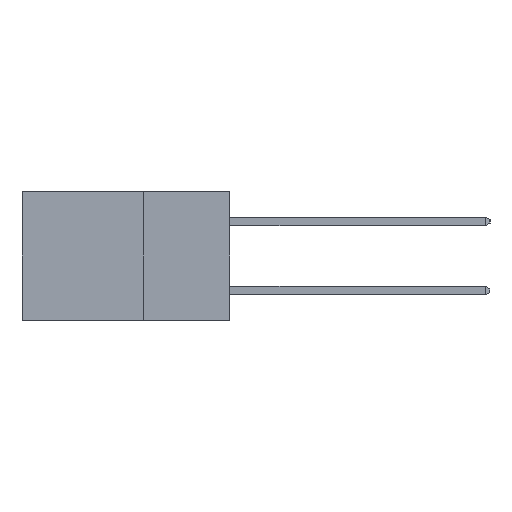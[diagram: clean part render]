
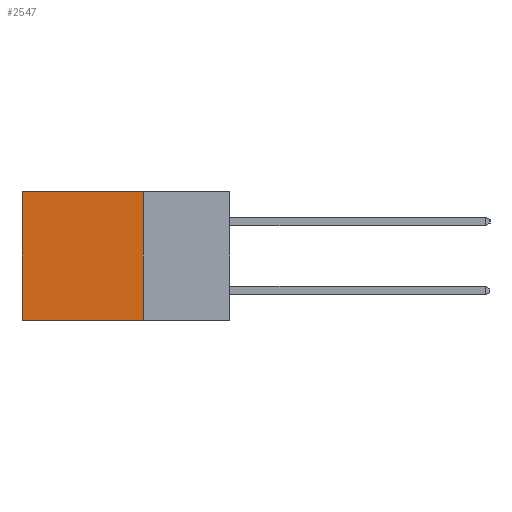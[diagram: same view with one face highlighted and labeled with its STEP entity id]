
A CAD part, left-side view. The second image highlights one B-rep face of the part: STEP entity #2547.
In plain terms, the highlighted planar face has unit normal (-1, 0, 0).
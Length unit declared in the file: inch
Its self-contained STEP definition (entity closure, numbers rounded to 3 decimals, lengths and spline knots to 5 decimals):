
#412 = DIRECTION ( 'NONE',  ( 0., 1., 0. ) ) ;
#1767 = CARTESIAN_POINT ( 'NONE',  ( 0.298, 0.25, -0.37 ) ) ;
#2547 = ADVANCED_FACE ( 'NONE', ( #4131 ), #16374, .F. ) ;
#2665 = VECTOR ( 'NONE', #412, 39.37008 ) ;
#3336 = CARTESIAN_POINT ( 'NONE',  ( 0.298, 0.6, 0. ) ) ;
#4131 = FACE_OUTER_BOUND ( 'NONE', #14093, .T. ) ;
#4266 = ORIENTED_EDGE ( 'NONE', *, *, #10154, .F. ) ;
#4810 = CARTESIAN_POINT ( 'NONE',  ( 0.298, 0.25, 0. ) ) ;
#6066 = CARTESIAN_POINT ( 'NONE',  ( 0.298, 0.25, 0. ) ) ;
#6399 = VECTOR ( 'NONE', #10143, 39.37008 ) ;
#7967 = VERTEX_POINT ( 'NONE', #12733 ) ;
#7995 = EDGE_CURVE ( 'NONE', #12291, #7967, #13401, .T. ) ;
#8408 = VERTEX_POINT ( 'NONE', #1767 ) ;
#8548 = EDGE_CURVE ( 'NONE', #12291, #8408, #15572, .T. ) ;
#8685 = VECTOR ( 'NONE', #11165, 39.37008 ) ;
#8904 = ORIENTED_EDGE ( 'NONE', *, *, #12904, .T. ) ;
#8967 = AXIS2_PLACEMENT_3D ( 'NONE', #15702, #15741, #15924 ) ;
#9699 = LINE ( 'NONE', #10950, #2665 ) ;
#10143 = DIRECTION ( 'NONE',  ( 0., 1., 0. ) ) ;
#10154 = EDGE_CURVE ( 'NONE', #8408, #13472, #9699, .T. ) ;
#10403 = ORIENTED_EDGE ( 'NONE', *, *, #7995, .T. ) ;
#10950 = CARTESIAN_POINT ( 'NONE',  ( 0.298, 0.25, -0.37 ) ) ;
#11165 = DIRECTION ( 'NONE',  ( 0., 0., -1. ) ) ;
#11221 = CARTESIAN_POINT ( 'NONE',  ( 0.298, 0.25, 0. ) ) ;
#11287 = LINE ( 'NONE', #3336, #14283 ) ;
#12291 = VERTEX_POINT ( 'NONE', #6066 ) ;
#12733 = CARTESIAN_POINT ( 'NONE',  ( 0.298, 0.6, 0. ) ) ;
#12904 = EDGE_CURVE ( 'NONE', #7967, #13472, #11287, .T. ) ;
#13401 = LINE ( 'NONE', #4810, #6399 ) ;
#13472 = VERTEX_POINT ( 'NONE', #15727 ) ;
#14093 = EDGE_LOOP ( 'NONE', ( #8904, #4266, #15820, #10403 ) ) ;
#14283 = VECTOR ( 'NONE', #15123, 39.37008 ) ;
#15123 = DIRECTION ( 'NONE',  ( 0., 0., -1. ) ) ;
#15572 = LINE ( 'NONE', #11221, #8685 ) ;
#15702 = CARTESIAN_POINT ( 'NONE',  ( 0.298, 0.25, 0. ) ) ;
#15727 = CARTESIAN_POINT ( 'NONE',  ( 0.298, 0.6, -0.37 ) ) ;
#15741 = DIRECTION ( 'NONE',  ( 1., 0., 0. ) ) ;
#15820 = ORIENTED_EDGE ( 'NONE', *, *, #8548, .F. ) ;
#15924 = DIRECTION ( 'NONE',  ( 0., 0., -1. ) ) ;
#16374 = PLANE ( 'NONE',  #8967 ) ;
